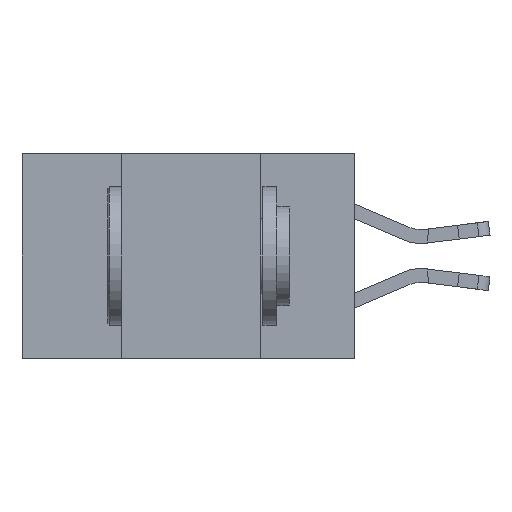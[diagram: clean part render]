
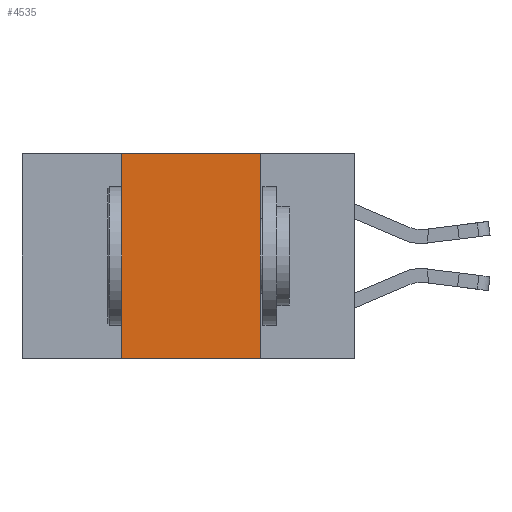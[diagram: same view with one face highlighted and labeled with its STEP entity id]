
A CAD part, left-side view. The second image highlights one B-rep face of the part: STEP entity #4535.
In plain terms, the highlighted planar face has unit normal (-1, 0, 0).
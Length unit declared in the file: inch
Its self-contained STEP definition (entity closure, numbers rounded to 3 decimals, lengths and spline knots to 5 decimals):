
#5 = VERTEX_POINT ( 'NONE', #17687 ) ;
#140 = DIRECTION ( 'NONE',  ( 0., -1., 0. ) ) ;
#2287 = LINE ( 'NONE', #13320, #10168 ) ;
#2483 = VERTEX_POINT ( 'NONE', #15695 ) ;
#2650 = VERTEX_POINT ( 'NONE', #4560 ) ;
#3052 = ORIENTED_EDGE ( 'NONE', *, *, #5660, .F. ) ;
#4535 = ADVANCED_FACE ( 'NONE', ( #6053 ), #16584, .F. ) ;
#4542 = EDGE_CURVE ( 'NONE', #2650, #5, #5067, .T. ) ;
#4560 = CARTESIAN_POINT ( 'NONE',  ( 0., 0.42, 0. ) ) ;
#4837 = LINE ( 'NONE', #5342, #10838 ) ;
#5067 = LINE ( 'NONE', #16738, #8619 ) ;
#5342 = CARTESIAN_POINT ( 'NONE',  ( 0., 0.17, 0. ) ) ;
#5507 = EDGE_CURVE ( 'NONE', #5, #12949, #4837, .T. ) ;
#5660 = EDGE_CURVE ( 'NONE', #2483, #2650, #9504, .T. ) ;
#6053 = FACE_OUTER_BOUND ( 'NONE', #18063, .T. ) ;
#6609 = ORIENTED_EDGE ( 'NONE', *, *, #4542, .F. ) ;
#8527 = DIRECTION ( 'NONE',  ( 0., 0., 1. ) ) ;
#8605 = VECTOR ( 'NONE', #8527, 39.37008 ) ;
#8619 = VECTOR ( 'NONE', #16632, 39.37008 ) ;
#9504 = LINE ( 'NONE', #18259, #8605 ) ;
#9856 = CARTESIAN_POINT ( 'NONE',  ( 0., 0.17, -0.37 ) ) ;
#10168 = VECTOR ( 'NONE', #140, 39.37008 ) ;
#10838 = VECTOR ( 'NONE', #18565, 39.37008 ) ;
#12949 = VERTEX_POINT ( 'NONE', #9856 ) ;
#13320 = CARTESIAN_POINT ( 'NONE',  ( 0., 0.6, -0.37 ) ) ;
#13689 = AXIS2_PLACEMENT_3D ( 'NONE', #15531, #17153, #16629 ) ;
#15081 = EDGE_CURVE ( 'NONE', #2483, #12949, #2287, .T. ) ;
#15313 = ORIENTED_EDGE ( 'NONE', *, *, #15081, .T. ) ;
#15531 = CARTESIAN_POINT ( 'NONE',  ( 0., 0.6, 0. ) ) ;
#15695 = CARTESIAN_POINT ( 'NONE',  ( 0., 0.42, -0.37 ) ) ;
#16584 = PLANE ( 'NONE',  #13689 ) ;
#16629 = DIRECTION ( 'NONE',  ( 0., 0., -1. ) ) ;
#16632 = DIRECTION ( 'NONE',  ( 0., -1., 0. ) ) ;
#16738 = CARTESIAN_POINT ( 'NONE',  ( 0., 0.6, 0. ) ) ;
#17153 = DIRECTION ( 'NONE',  ( 1., 0., 0. ) ) ;
#17271 = ORIENTED_EDGE ( 'NONE', *, *, #5507, .F. ) ;
#17687 = CARTESIAN_POINT ( 'NONE',  ( 0., 0.17, 0. ) ) ;
#18063 = EDGE_LOOP ( 'NONE', ( #17271, #6609, #3052, #15313 ) ) ;
#18259 = CARTESIAN_POINT ( 'NONE',  ( 0., 0.42, 0. ) ) ;
#18565 = DIRECTION ( 'NONE',  ( 0., 0., -1. ) ) ;
